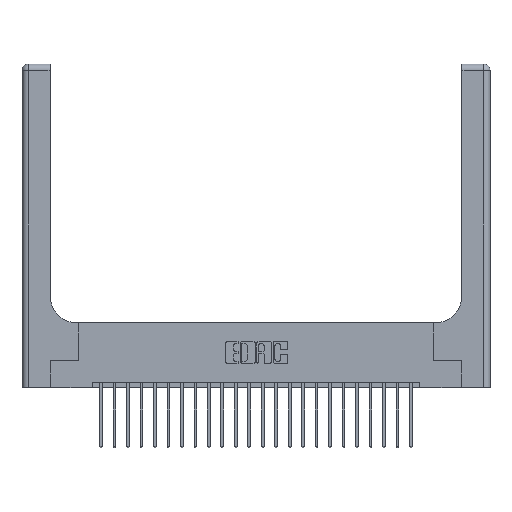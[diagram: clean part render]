
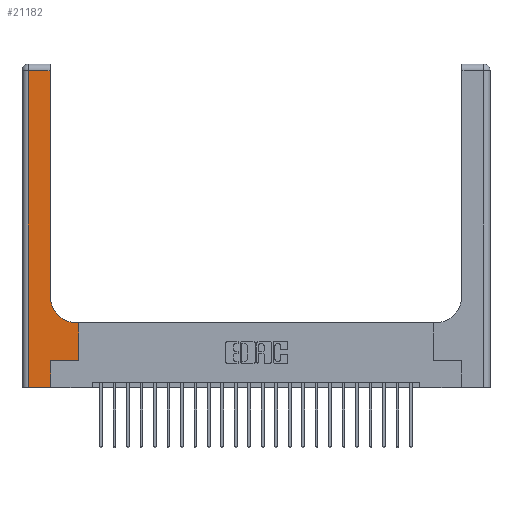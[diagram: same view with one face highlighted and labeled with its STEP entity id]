
A CAD part, top view. The second image highlights one B-rep face of the part: STEP entity #21182.
In plain terms, the highlighted planar face has unit normal (0, 0, 1).
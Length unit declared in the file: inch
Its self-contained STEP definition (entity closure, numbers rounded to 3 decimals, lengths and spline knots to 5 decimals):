
#9 = LINE ( 'NONE', #17906, #18570 ) ;
#448 = DIRECTION ( 'NONE',  ( -1., 0., 0. ) ) ;
#525 = CARTESIAN_POINT ( 'NONE',  ( 0.26, 3., 0.37 ) ) ;
#688 = EDGE_CURVE ( 'NONE', #3701, #14539, #3323, .T. ) ;
#959 = EDGE_LOOP ( 'NONE', ( #12067, #20530, #12910, #22770, #8717, #17394, #9258, #18799, #18566 ) ) ;
#1589 = VERTEX_POINT ( 'NONE', #4865 ) ;
#1746 = EDGE_CURVE ( 'NONE', #15065, #16854, #20836, .T. ) ;
#2475 = EDGE_CURVE ( 'NONE', #1589, #3701, #22508, .T. ) ;
#2488 = DIRECTION ( 'NONE',  ( 0., 1., 0. ) ) ;
#3323 = CIRCLE ( 'NONE', #13082, 0.25 ) ;
#3471 = CARTESIAN_POINT ( 'NONE',  ( 0.265, 0., 0.37 ) ) ;
#3613 = DIRECTION ( 'NONE',  ( 0., 1., 0. ) ) ;
#3701 = VERTEX_POINT ( 'NONE', #7257 ) ;
#3855 = CARTESIAN_POINT ( 'NONE',  ( 0.26, 2.94, 0.37 ) ) ;
#4152 = VECTOR ( 'NONE', #19575, 39.37008 ) ;
#4865 = CARTESIAN_POINT ( 'NONE',  ( 0.528, 0.6, 0.37 ) ) ;
#5169 = CARTESIAN_POINT ( 'NONE',  ( 0.26, 0.85, 0.37 ) ) ;
#5342 = FACE_OUTER_BOUND ( 'NONE', #959, .T. ) ;
#5455 = AXIS2_PLACEMENT_3D ( 'NONE', #15262, #8085, #9644 ) ;
#6003 = DIRECTION ( 'NONE',  ( 1., 0., 0. ) ) ;
#6048 = LINE ( 'NONE', #525, #12829 ) ;
#6244 = DIRECTION ( 'NONE',  ( 0., -1., 0. ) ) ;
#6602 = CARTESIAN_POINT ( 'NONE',  ( 0.06, 0., 0.37 ) ) ;
#7252 = VERTEX_POINT ( 'NONE', #19785 ) ;
#7257 = CARTESIAN_POINT ( 'NONE',  ( 0.51, 0.6, 0.37 ) ) ;
#7755 = DIRECTION ( 'NONE',  ( 1., 0., 0. ) ) ;
#7980 = CARTESIAN_POINT ( 'NONE',  ( 0., 0., 0.37 ) ) ;
#8085 = DIRECTION ( 'NONE',  ( 0., 0., -1. ) ) ;
#8717 = ORIENTED_EDGE ( 'NONE', *, *, #14626, .T. ) ;
#8756 = CARTESIAN_POINT ( 'NONE',  ( 0.528, 0.25, 0.37 ) ) ;
#9258 = ORIENTED_EDGE ( 'NONE', *, *, #14350, .T. ) ;
#9644 = DIRECTION ( 'NONE',  ( -1., 0., 0. ) ) ;
#9902 = CARTESIAN_POINT ( 'NONE',  ( 0.265, 0., 0.37 ) ) ;
#10084 = CARTESIAN_POINT ( 'NONE',  ( 0.26, 0.6, 0.37 ) ) ;
#10133 = VERTEX_POINT ( 'NONE', #3855 ) ;
#10363 = LINE ( 'NONE', #3471, #10909 ) ;
#10829 = LINE ( 'NONE', #22450, #13406 ) ;
#10909 = VECTOR ( 'NONE', #3613, 39.37008 ) ;
#12067 = ORIENTED_EDGE ( 'NONE', *, *, #12992, .T. ) ;
#12267 = CARTESIAN_POINT ( 'NONE',  ( 0.265, 0.25, 0.37 ) ) ;
#12829 = VECTOR ( 'NONE', #2488, 39.37008 ) ;
#12910 = ORIENTED_EDGE ( 'NONE', *, *, #16182, .T. ) ;
#12992 = EDGE_CURVE ( 'NONE', #14539, #10133, #6048, .T. ) ;
#13082 = AXIS2_PLACEMENT_3D ( 'NONE', #13341, #18439, #7755 ) ;
#13208 = PLANE ( 'NONE',  #5455 ) ;
#13341 = CARTESIAN_POINT ( 'NONE',  ( 0.51, 0.85, 0.37 ) ) ;
#13406 = VECTOR ( 'NONE', #6244, 39.37008 ) ;
#14104 = VERTEX_POINT ( 'NONE', #16493 ) ;
#14350 = EDGE_CURVE ( 'NONE', #16959, #1589, #19681, .T. ) ;
#14539 = VERTEX_POINT ( 'NONE', #5169 ) ;
#14626 = EDGE_CURVE ( 'NONE', #16854, #14104, #10363, .T. ) ;
#14883 = LINE ( 'NONE', #12267, #4152 ) ;
#14911 = VECTOR ( 'NONE', #20191, 39.37008 ) ;
#15065 = VERTEX_POINT ( 'NONE', #6602 ) ;
#15141 = EDGE_CURVE ( 'NONE', #14104, #16959, #14883, .T. ) ;
#15262 = CARTESIAN_POINT ( 'NONE',  ( 0., 3., 0.37 ) ) ;
#15630 = DIRECTION ( 'NONE',  ( -1., 0., 0. ) ) ;
#16182 = EDGE_CURVE ( 'NONE', #7252, #15065, #10829, .T. ) ;
#16493 = CARTESIAN_POINT ( 'NONE',  ( 0.265, 0.25, 0.37 ) ) ;
#16854 = VERTEX_POINT ( 'NONE', #9902 ) ;
#16959 = VERTEX_POINT ( 'NONE', #8756 ) ;
#17394 = ORIENTED_EDGE ( 'NONE', *, *, #15141, .T. ) ;
#17906 = CARTESIAN_POINT ( 'NONE',  ( 0., 2.94, 0.37 ) ) ;
#18439 = DIRECTION ( 'NONE',  ( 0., 0., -1. ) ) ;
#18566 = ORIENTED_EDGE ( 'NONE', *, *, #688, .T. ) ;
#18570 = VECTOR ( 'NONE', #448, 39.37008 ) ;
#18799 = ORIENTED_EDGE ( 'NONE', *, *, #2475, .T. ) ;
#19575 = DIRECTION ( 'NONE',  ( 1., 0., 0. ) ) ;
#19681 = LINE ( 'NONE', #20115, #14911 ) ;
#19785 = CARTESIAN_POINT ( 'NONE',  ( 0.06, 2.94, 0.37 ) ) ;
#20115 = CARTESIAN_POINT ( 'NONE',  ( 0.528, 0.25, 0.37 ) ) ;
#20191 = DIRECTION ( 'NONE',  ( 0., 1., 0. ) ) ;
#20277 = VECTOR ( 'NONE', #6003, 39.37008 ) ;
#20530 = ORIENTED_EDGE ( 'NONE', *, *, #20899, .T. ) ;
#20836 = LINE ( 'NONE', #7980, #20277 ) ;
#20899 = EDGE_CURVE ( 'NONE', #10133, #7252, #9, .T. ) ;
#21182 = ADVANCED_FACE ( 'NONE', ( #5342 ), #13208, .F. ) ;
#21941 = VECTOR ( 'NONE', #15630, 39.37008 ) ;
#22450 = CARTESIAN_POINT ( 'NONE',  ( 0.06, 3., 0.37 ) ) ;
#22508 = LINE ( 'NONE', #10084, #21941 ) ;
#22770 = ORIENTED_EDGE ( 'NONE', *, *, #1746, .T. ) ;
